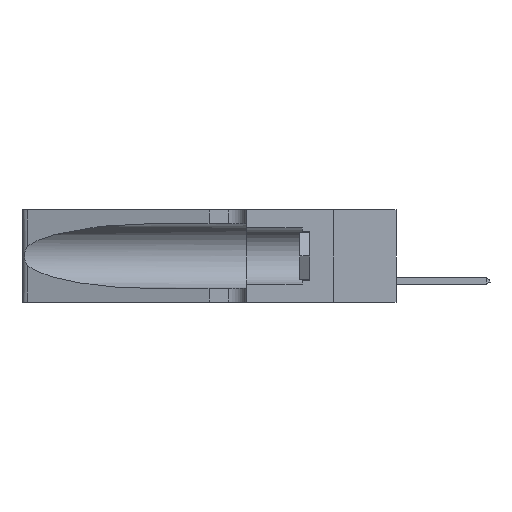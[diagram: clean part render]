
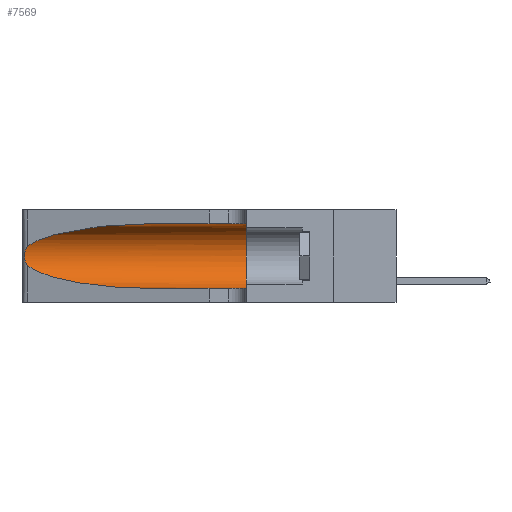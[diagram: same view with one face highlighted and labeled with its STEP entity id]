
A CAD part, left-side view. The second image highlights one B-rep face of the part: STEP entity #7569.
In plain terms, the highlighted cylindrical face has radius 3.308 mm (diameter 6.617 mm), a partial arc.
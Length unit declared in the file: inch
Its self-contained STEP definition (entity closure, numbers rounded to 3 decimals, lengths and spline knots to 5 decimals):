
#272 =( BOUNDED_CURVE ( )  B_SPLINE_CURVE ( 3, ( #21586, #35810, #18321, #42971 ),
 .UNSPECIFIED., .F., .F. ) 
 B_SPLINE_CURVE_WITH_KNOTS ( ( 4, 4 ),
 ( 1.5708, 2.84003 ),
 .UNSPECIFIED. ) 
 CURVE ( )  GEOMETRIC_REPRESENTATION_ITEM ( )  RATIONAL_B_SPLINE_CURVE ( ( 1., 0.87, 0.87, 1. ) ) 
 REPRESENTATION_ITEM ( '' )  );
#298 = AXIS2_PLACEMENT_3D ( 'NONE', #38075, #34926, #3979 ) ;
#901 = FACE_OUTER_BOUND ( 'NONE', #1143, .T. ) ;
#1143 = EDGE_LOOP ( 'NONE', ( #43827, #27578, #19684, #27789, #12159, #5704 ) ) ;
#2013 = EDGE_CURVE ( 'NONE', #39261, #17749, #272, .T. ) ;
#3296 = CARTESIAN_POINT ( 'NONE',  ( 0.1305, 1.61858, 0.31525 ) ) ;
#3979 = DIRECTION ( 'NONE',  ( 0., 0., -1. ) ) ;
#5704 = ORIENTED_EDGE ( 'NONE', *, *, #39463, .F. ) ;
#6127 = CARTESIAN_POINT ( 'NONE',  ( 0.26075, 1.23896, 0.19203 ) ) ;
#6422 = CARTESIAN_POINT ( 'NONE',  ( 0.25555, 1.22993, 0.14849 ) ) ;
#6925 = VECTOR ( 'NONE', #14235, 39.37008 ) ;
#7569 = ADVANCED_FACE ( 'NONE', ( #901 ), #31380, .F. ) ;
#7645 = VERTEX_POINT ( 'NONE', #42202 ) ;
#7859 = CARTESIAN_POINT ( 'NONE',  ( 0.1305, 0.35, 0.31525 ) ) ;
#8022 = VERTEX_POINT ( 'NONE', #22299 ) ;
#8792 = CARTESIAN_POINT ( 'NONE',  ( 0.25555, 1.22994, 0.2215 ) ) ;
#10734 = EDGE_CURVE ( 'NONE', #17749, #12365, #37260, .T. ) ;
#11728 = CARTESIAN_POINT ( 'NONE',  ( 0.25487, 1.22718, 0.14631 ) ) ;
#12159 = ORIENTED_EDGE ( 'NONE', *, *, #13246, .F. ) ;
#12261 = CARTESIAN_POINT ( 'NONE',  ( 0.25487, 1.22718, 0.14631 ) ) ;
#12365 = VERTEX_POINT ( 'NONE', #12261 ) ;
#13020 = CARTESIAN_POINT ( 'NONE',  ( 0.25854, 1.2359, 0.20912 ) ) ;
#13168 = CARTESIAN_POINT ( 'NONE',  ( 0.26075, 1.23896, 0.178 ) ) ;
#13246 = EDGE_CURVE ( 'NONE', #20507, #8022, #42927, .T. ) ;
#13381 = DIRECTION ( 'NONE',  ( 0., -1., 0. ) ) ;
#14235 = DIRECTION ( 'NONE',  ( 0., -1., 0. ) ) ;
#14804 =( BOUNDED_CURVE ( )  B_SPLINE_CURVE ( 3, ( #11728, #39121, #32101, #21889 ),
 .UNSPECIFIED., .F., .F. ) 
 B_SPLINE_CURVE_WITH_KNOTS ( ( 4, 4 ),
 ( 3.44316, 4.71239 ),
 .UNSPECIFIED. ) 
 CURVE ( )  GEOMETRIC_REPRESENTATION_ITEM ( )  RATIONAL_B_SPLINE_CURVE ( ( 1., 0.87, 0.87, 1. ) ) 
 REPRESENTATION_ITEM ( '' )  );
#17749 = VERTEX_POINT ( 'NONE', #27919 ) ;
#18321 = CARTESIAN_POINT ( 'NONE',  ( 0.2373, 1.15595, 0.28018 ) ) ;
#18827 = VECTOR ( 'NONE', #13381, 39.37008 ) ;
#19011 = CARTESIAN_POINT ( 'NONE',  ( 0.25487, 1.22718, 0.22369 ) ) ;
#19149 = CARTESIAN_POINT ( 'NONE',  ( 0.25787, 1.23484, 0.2124 ) ) ;
#19684 = ORIENTED_EDGE ( 'NONE', *, *, #27165, .T. ) ;
#19877 = CARTESIAN_POINT ( 'NONE',  ( 0.25789, 1.23486, 0.15765 ) ) ;
#20507 = VERTEX_POINT ( 'NONE', #7859 ) ;
#21586 = CARTESIAN_POINT ( 'NONE',  ( 0.1305, 0.72297, 0.31525 ) ) ;
#21889 = CARTESIAN_POINT ( 'NONE',  ( 0.1305, 0.72297, 0.05475 ) ) ;
#21905 = LINE ( 'NONE', #3296, #6925 ) ;
#22299 = CARTESIAN_POINT ( 'NONE',  ( 0.1305, 0.35, 0.05475 ) ) ;
#22541 = LINE ( 'NONE', #30282, #18827 ) ;
#22715 = CARTESIAN_POINT ( 'NONE',  ( 0.1305, 0.72297, 0.31525 ) ) ;
#26604 = CARTESIAN_POINT ( 'NONE',  ( 0.26017, 1.23833, 0.17102 ) ) ;
#27165 = EDGE_CURVE ( 'NONE', #12365, #7645, #14804, .T. ) ;
#27578 = ORIENTED_EDGE ( 'NONE', *, *, #10734, .T. ) ;
#27789 = ORIENTED_EDGE ( 'NONE', *, *, #32522, .T. ) ;
#27919 = CARTESIAN_POINT ( 'NONE',  ( 0.25487, 1.22718, 0.22369 ) ) ;
#30282 = CARTESIAN_POINT ( 'NONE',  ( 0.1305, 1.61858, 0.05475 ) ) ;
#30454 = DIRECTION ( 'NONE',  ( 0., 0., 1. ) ) ;
#31380 = CYLINDRICAL_SURFACE ( 'NONE', #298, 0.13025 ) ;
#32101 = CARTESIAN_POINT ( 'NONE',  ( 0.18966, 0.96281, 0.05475 ) ) ;
#32522 = EDGE_CURVE ( 'NONE', #7645, #8022, #22541, .T. ) ;
#33380 = CARTESIAN_POINT ( 'NONE',  ( 0.25856, 1.23593, 0.16098 ) ) ;
#33617 = CARTESIAN_POINT ( 'NONE',  ( 0.1305, 0.35, 0.185 ) ) ;
#34926 = DIRECTION ( 'NONE',  ( 0., -1., 0. ) ) ;
#35810 = CARTESIAN_POINT ( 'NONE',  ( 0.18966, 0.96281, 0.31525 ) ) ;
#36949 = CARTESIAN_POINT ( 'NONE',  ( 0.25639, 1.23186, 0.15144 ) ) ;
#37039 = DIRECTION ( 'NONE',  ( 0., 1., 0. ) ) ;
#37260 = B_SPLINE_CURVE_WITH_KNOTS ( 'NONE', 3,
 ( #19011, #8792, #42949, #19149, #13020, #40414, #6127, #13168, #26604, #33380, #19877, #36949, #6422, #40253 ),
 .UNSPECIFIED., .F., .F.,
 ( 4, 2, 2, 2, 2, 2, 4 ),
 ( 0., 0.00027, 0.00053, 0.00107, 0.0016, 0.00187, 0.00214 ),
 .UNSPECIFIED. ) ;
#37706 = AXIS2_PLACEMENT_3D ( 'NONE', #33617, #37039, #30454 ) ;
#38075 = CARTESIAN_POINT ( 'NONE',  ( 0.1305, 1.61858, 0.185 ) ) ;
#39121 = CARTESIAN_POINT ( 'NONE',  ( 0.2373, 1.15595, 0.08982 ) ) ;
#39261 = VERTEX_POINT ( 'NONE', #22715 ) ;
#39463 = EDGE_CURVE ( 'NONE', #39261, #20507, #21905, .T. ) ;
#40253 = CARTESIAN_POINT ( 'NONE',  ( 0.25487, 1.22718, 0.14631 ) ) ;
#40414 = CARTESIAN_POINT ( 'NONE',  ( 0.26018, 1.23835, 0.19895 ) ) ;
#42202 = CARTESIAN_POINT ( 'NONE',  ( 0.1305, 0.72297, 0.05475 ) ) ;
#42927 = CIRCLE ( 'NONE', #37706, 0.13025 ) ;
#42949 = CARTESIAN_POINT ( 'NONE',  ( 0.25639, 1.23184, 0.21858 ) ) ;
#42971 = CARTESIAN_POINT ( 'NONE',  ( 0.25487, 1.22718, 0.22369 ) ) ;
#43827 = ORIENTED_EDGE ( 'NONE', *, *, #2013, .T. ) ;
